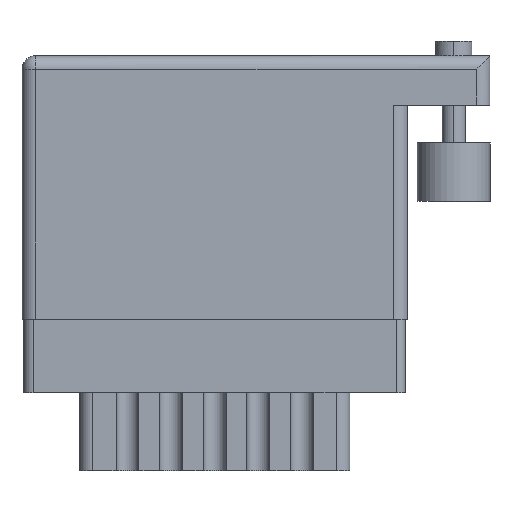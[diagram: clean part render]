
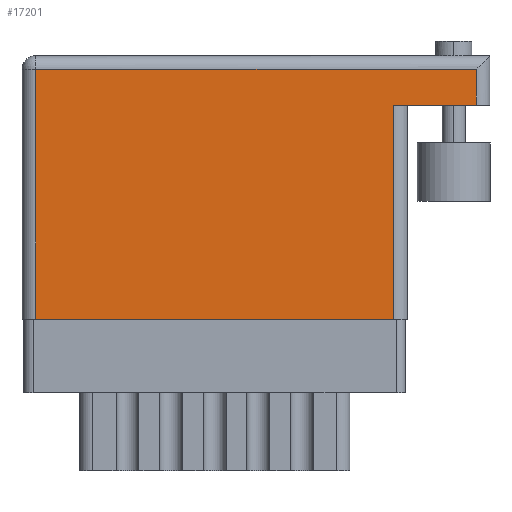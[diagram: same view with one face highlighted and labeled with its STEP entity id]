
A CAD part, front view. The second image highlights one B-rep face of the part: STEP entity #17201.
In plain terms, the highlighted face is planar.
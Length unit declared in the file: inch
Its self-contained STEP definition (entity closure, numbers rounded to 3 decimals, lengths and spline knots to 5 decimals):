
#301 = LINE ( 'NONE', #12307, #14143 ) ;
#1389 = VECTOR ( 'NONE', #8387, 39.37008 ) ;
#1817 = EDGE_CURVE ( 'NONE', #16820, #10850, #23155, .T. ) ;
#2153 = ORIENTED_EDGE ( 'NONE', *, *, #23944, .T. ) ;
#2922 = DIRECTION ( 'NONE',  ( -1., 0., 0. ) ) ;
#3515 = VERTEX_POINT ( 'NONE', #11744 ) ;
#3572 = LINE ( 'NONE', #11393, #20955 ) ;
#4487 = EDGE_CURVE ( 'NONE', #3515, #11548, #25707, .T. ) ;
#5995 = VERTEX_POINT ( 'NONE', #20269 ) ;
#6199 = CARTESIAN_POINT ( 'NONE',  ( 0.047, 0.859, 0. ) ) ;
#6415 = ORIENTED_EDGE ( 'NONE', *, *, #17079, .T. ) ;
#7617 = EDGE_CURVE ( 'NONE', #13384, #3515, #301, .T. ) ;
#7882 = CARTESIAN_POINT ( 'NONE',  ( 0., 0.859, 0. ) ) ;
#8387 = DIRECTION ( 'NONE',  ( -1., 0., 0. ) ) ;
#8632 = DIRECTION ( 'NONE',  ( 1., 0., 0. ) ) ;
#10581 = VECTOR ( 'NONE', #8632, 39.37008 ) ;
#10850 = VERTEX_POINT ( 'NONE', #24427 ) ;
#11393 = CARTESIAN_POINT ( 'NONE',  ( 1.278, 0.736, 0. ) ) ;
#11548 = VERTEX_POINT ( 'NONE', #6199 ) ;
#11744 = CARTESIAN_POINT ( 'NONE',  ( 1.562, 0.859, 0. ) ) ;
#12307 = CARTESIAN_POINT ( 'NONE',  ( 1.562, 0.906, 0. ) ) ;
#12824 = CARTESIAN_POINT ( 'NONE',  ( 0., 0.906, 0. ) ) ;
#13278 = VECTOR ( 'NONE', #18812, 39.37008 ) ;
#13338 = ORIENTED_EDGE ( 'NONE', *, *, #21527, .F. ) ;
#13384 = VERTEX_POINT ( 'NONE', #17263 ) ;
#14143 = VECTOR ( 'NONE', #19978, 39.37008 ) ;
#14943 = AXIS2_PLACEMENT_3D ( 'NONE', #12824, #25269, #2922 ) ;
#15730 = ORIENTED_EDGE ( 'NONE', *, *, #7617, .T. ) ;
#15839 = DIRECTION ( 'NONE',  ( -1., 0., 0. ) ) ;
#16491 = LINE ( 'NONE', #22570, #1389 ) ;
#16820 = VERTEX_POINT ( 'NONE', #21664 ) ;
#17079 = EDGE_CURVE ( 'NONE', #11548, #16820, #21243, .T. ) ;
#17201 = ADVANCED_FACE ( 'NONE', ( #19189 ), #20743, .F. ) ;
#17263 = CARTESIAN_POINT ( 'NONE',  ( 1.562, 0.736, 0. ) ) ;
#17339 = ORIENTED_EDGE ( 'NONE', *, *, #4487, .T. ) ;
#18548 = CARTESIAN_POINT ( 'NONE',  ( 0., 0., 0. ) ) ;
#18812 = DIRECTION ( 'NONE',  ( 0., -1., 0. ) ) ;
#19189 = FACE_OUTER_BOUND ( 'NONE', #25705, .T. ) ;
#19581 = DIRECTION ( 'NONE',  ( 0., 1., 0. ) ) ;
#19978 = DIRECTION ( 'NONE',  ( 0., 1., 0. ) ) ;
#20056 = ORIENTED_EDGE ( 'NONE', *, *, #1817, .T. ) ;
#20269 = CARTESIAN_POINT ( 'NONE',  ( 1.278, 0.736, 0. ) ) ;
#20743 = PLANE ( 'NONE',  #14943 ) ;
#20955 = VECTOR ( 'NONE', #19581, 39.37008 ) ;
#21118 = CARTESIAN_POINT ( 'NONE',  ( 0.047, 0., 0. ) ) ;
#21243 = LINE ( 'NONE', #21118, #13278 ) ;
#21527 = EDGE_CURVE ( 'NONE', #13384, #5995, #16491, .T. ) ;
#21664 = CARTESIAN_POINT ( 'NONE',  ( 0.047, 0., 0. ) ) ;
#22570 = CARTESIAN_POINT ( 'NONE',  ( 1.609, 0.736, 0. ) ) ;
#23155 = LINE ( 'NONE', #18548, #10581 ) ;
#23466 = VECTOR ( 'NONE', #15839, 39.37008 ) ;
#23944 = EDGE_CURVE ( 'NONE', #10850, #5995, #3572, .T. ) ;
#24427 = CARTESIAN_POINT ( 'NONE',  ( 1.278, 0., 0. ) ) ;
#25269 = DIRECTION ( 'NONE',  ( 0., 0., -1. ) ) ;
#25705 = EDGE_LOOP ( 'NONE', ( #20056, #2153, #13338, #15730, #17339, #6415 ) ) ;
#25707 = LINE ( 'NONE', #7882, #23466 ) ;
